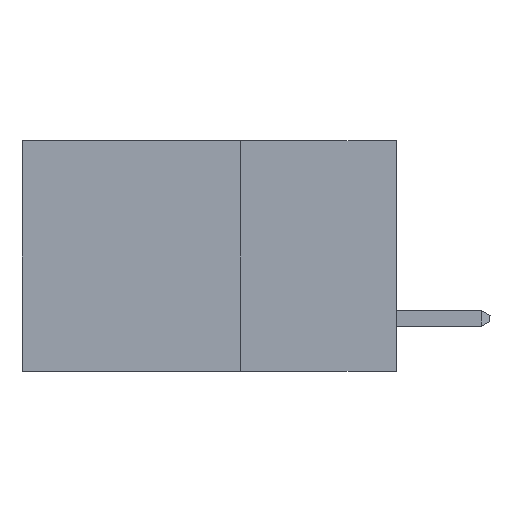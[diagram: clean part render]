
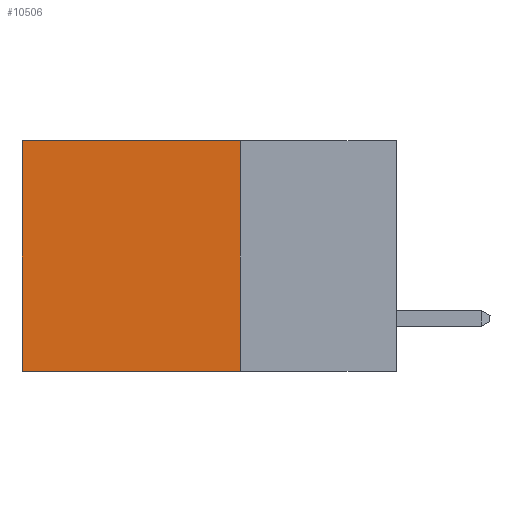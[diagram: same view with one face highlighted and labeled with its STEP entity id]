
A CAD part, left-side view. The second image highlights one B-rep face of the part: STEP entity #10506.
In plain terms, the highlighted planar face has unit normal (-1, 0, 0).
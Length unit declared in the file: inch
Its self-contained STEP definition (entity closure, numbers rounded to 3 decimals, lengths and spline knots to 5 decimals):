
#584 = VERTEX_POINT ( 'NONE', #3118 ) ;
#1302 = CARTESIAN_POINT ( 'NONE',  ( 0.2615, 0.25, -0.37 ) ) ;
#1354 = DIRECTION ( 'NONE',  ( 0., 1., 0. ) ) ;
#1574 = VERTEX_POINT ( 'NONE', #8697 ) ;
#1758 = EDGE_CURVE ( 'NONE', #12353, #584, #12179, .T. ) ;
#2641 = DIRECTION ( 'NONE',  ( 0., 0., -1. ) ) ;
#2745 = PLANE ( 'NONE',  #10923 ) ;
#2752 = CARTESIAN_POINT ( 'NONE',  ( 0.2615, 0.25, 0. ) ) ;
#2845 = CARTESIAN_POINT ( 'NONE',  ( 0.2615, 0.25, -0.37 ) ) ;
#3118 = CARTESIAN_POINT ( 'NONE',  ( 0.2615, 0.25, -0.37 ) ) ;
#3516 = DIRECTION ( 'NONE',  ( 0., 0., -1. ) ) ;
#3719 = EDGE_LOOP ( 'NONE', ( #3774, #5957, #5789, #4052 ) ) ;
#3774 = ORIENTED_EDGE ( 'NONE', *, *, #5585, .T. ) ;
#3975 = DIRECTION ( 'NONE',  ( 1., 0., 0. ) ) ;
#4052 = ORIENTED_EDGE ( 'NONE', *, *, #13391, .T. ) ;
#5088 = FACE_OUTER_BOUND ( 'NONE', #3719, .T. ) ;
#5379 = DIRECTION ( 'NONE',  ( 0., 1., 0. ) ) ;
#5585 = EDGE_CURVE ( 'NONE', #9178, #1574, #7182, .T. ) ;
#5789 = ORIENTED_EDGE ( 'NONE', *, *, #1758, .F. ) ;
#5957 = ORIENTED_EDGE ( 'NONE', *, *, #13764, .F. ) ;
#6433 = LINE ( 'NONE', #11105, #7878 ) ;
#7182 = LINE ( 'NONE', #11604, #13455 ) ;
#7878 = VECTOR ( 'NONE', #5379, 39.37008 ) ;
#8057 = DIRECTION ( 'NONE',  ( 0., 0., -1. ) ) ;
#8697 = CARTESIAN_POINT ( 'NONE',  ( 0.2615, 0.6, -0.37 ) ) ;
#9093 = CARTESIAN_POINT ( 'NONE',  ( 0.2615, 0.25, -0.37 ) ) ;
#9178 = VERTEX_POINT ( 'NONE', #11629 ) ;
#10506 = ADVANCED_FACE ( 'NONE', ( #5088 ), #2745, .F. ) ;
#10923 = AXIS2_PLACEMENT_3D ( 'NONE', #2845, #3975, #2641 ) ;
#11105 = CARTESIAN_POINT ( 'NONE',  ( 0.2615, 0.25, 0. ) ) ;
#11604 = CARTESIAN_POINT ( 'NONE',  ( 0.2615, 0.6, -0.37 ) ) ;
#11629 = CARTESIAN_POINT ( 'NONE',  ( 0.2615, 0.6, 0. ) ) ;
#12147 = VECTOR ( 'NONE', #1354, 39.37008 ) ;
#12179 = LINE ( 'NONE', #9093, #14178 ) ;
#12353 = VERTEX_POINT ( 'NONE', #2752 ) ;
#13391 = EDGE_CURVE ( 'NONE', #12353, #9178, #6433, .T. ) ;
#13455 = VECTOR ( 'NONE', #8057, 39.37008 ) ;
#13764 = EDGE_CURVE ( 'NONE', #584, #1574, #14698, .T. ) ;
#14178 = VECTOR ( 'NONE', #3516, 39.37008 ) ;
#14698 = LINE ( 'NONE', #1302, #12147 ) ;
